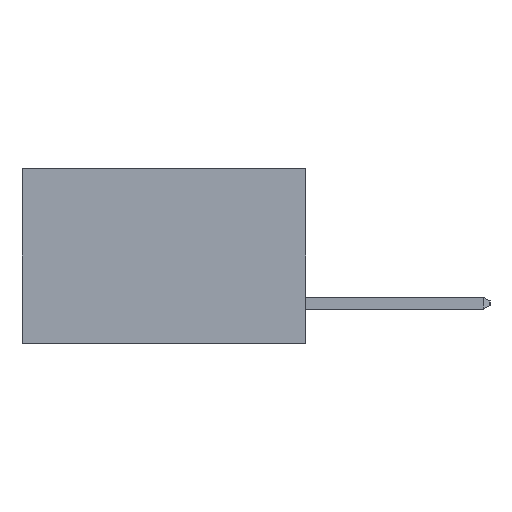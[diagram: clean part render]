
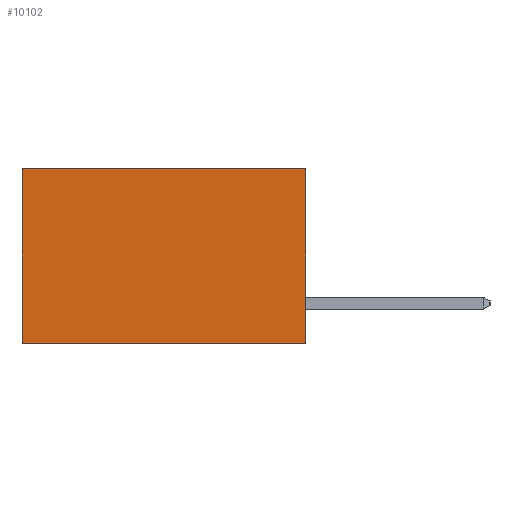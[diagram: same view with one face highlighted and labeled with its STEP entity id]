
A CAD part, left-side view. The second image highlights one B-rep face of the part: STEP entity #10102.
In plain terms, the highlighted planar face has unit normal (-1, 0, 0).
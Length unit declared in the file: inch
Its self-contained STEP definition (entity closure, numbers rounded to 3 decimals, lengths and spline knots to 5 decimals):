
#350 = VECTOR ( 'NONE', #6892, 39.37008 ) ;
#374 = VERTEX_POINT ( 'NONE', #1118 ) ;
#865 = LINE ( 'NONE', #9379, #350 ) ;
#1075 = DIRECTION ( 'NONE',  ( 0., 0., -1. ) ) ;
#1118 = CARTESIAN_POINT ( 'NONE',  ( 0.298, 0.6, -0.37 ) ) ;
#1255 = CARTESIAN_POINT ( 'NONE',  ( 0.298, 0., -0.37 ) ) ;
#1508 = LINE ( 'NONE', #5475, #5646 ) ;
#1513 = ORIENTED_EDGE ( 'NONE', *, *, #3865, .F. ) ;
#3067 = EDGE_CURVE ( 'NONE', #3407, #5803, #9570, .T. ) ;
#3407 = VERTEX_POINT ( 'NONE', #4217 ) ;
#3555 = DIRECTION ( 'NONE',  ( 1., 0., 0. ) ) ;
#3594 = CARTESIAN_POINT ( 'NONE',  ( 0.298, 0.6, 0. ) ) ;
#3686 = VECTOR ( 'NONE', #1075, 39.37008 ) ;
#3865 = EDGE_CURVE ( 'NONE', #5803, #374, #1508, .T. ) ;
#4010 = VERTEX_POINT ( 'NONE', #9824 ) ;
#4174 = CARTESIAN_POINT ( 'NONE',  ( 0.298, 0., 0. ) ) ;
#4217 = CARTESIAN_POINT ( 'NONE',  ( 0.298, 0., 0. ) ) ;
#4297 = AXIS2_PLACEMENT_3D ( 'NONE', #10089, #3555, #9298 ) ;
#4608 = DIRECTION ( 'NONE',  ( 0., 0., -1. ) ) ;
#5475 = CARTESIAN_POINT ( 'NONE',  ( 0.298, 0., -0.37 ) ) ;
#5646 = VECTOR ( 'NONE', #5652, 39.37008 ) ;
#5652 = DIRECTION ( 'NONE',  ( 0., 1., 0. ) ) ;
#5803 = VERTEX_POINT ( 'NONE', #1255 ) ;
#5821 = LINE ( 'NONE', #3594, #3686 ) ;
#6251 = EDGE_CURVE ( 'NONE', #4010, #374, #5821, .T. ) ;
#6530 = EDGE_LOOP ( 'NONE', ( #6591, #1513, #6602, #9799 ) ) ;
#6591 = ORIENTED_EDGE ( 'NONE', *, *, #6251, .T. ) ;
#6602 = ORIENTED_EDGE ( 'NONE', *, *, #3067, .F. ) ;
#6821 = PLANE ( 'NONE',  #4297 ) ;
#6892 = DIRECTION ( 'NONE',  ( 0., 1., 0. ) ) ;
#7929 = VECTOR ( 'NONE', #4608, 39.37008 ) ;
#8137 = EDGE_CURVE ( 'NONE', #3407, #4010, #865, .T. ) ;
#9298 = DIRECTION ( 'NONE',  ( 0., 0., -1. ) ) ;
#9379 = CARTESIAN_POINT ( 'NONE',  ( 0.298, 0., 0. ) ) ;
#9570 = LINE ( 'NONE', #4174, #7929 ) ;
#9799 = ORIENTED_EDGE ( 'NONE', *, *, #8137, .T. ) ;
#9824 = CARTESIAN_POINT ( 'NONE',  ( 0.298, 0.6, 0. ) ) ;
#10089 = CARTESIAN_POINT ( 'NONE',  ( 0.298, 0., 0. ) ) ;
#10102 = ADVANCED_FACE ( 'NONE', ( #10395 ), #6821, .F. ) ;
#10395 = FACE_OUTER_BOUND ( 'NONE', #6530, .T. ) ;
